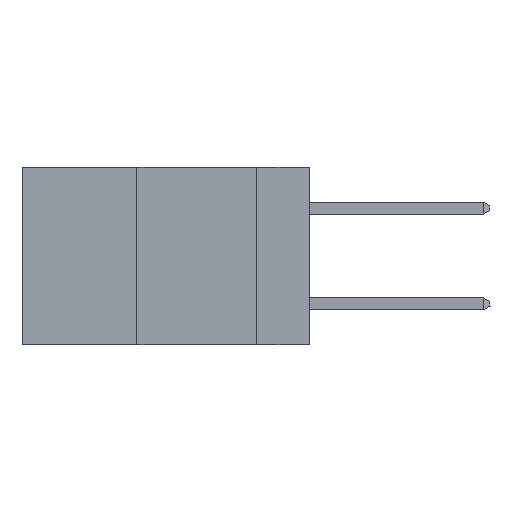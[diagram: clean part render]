
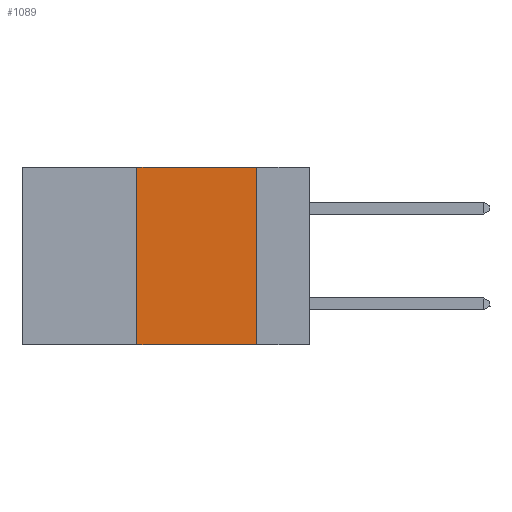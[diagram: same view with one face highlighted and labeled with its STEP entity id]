
A CAD part, left-side view. The second image highlights one B-rep face of the part: STEP entity #1089.
In plain terms, the highlighted planar face has unit normal (-1, 0, 0).
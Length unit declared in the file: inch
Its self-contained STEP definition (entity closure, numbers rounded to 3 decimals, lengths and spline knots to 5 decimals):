
#1089 = ADVANCED_FACE ( 'NONE', ( #18183 ), #6968, .F. ) ;
#2550 = DIRECTION ( 'NONE',  ( 0., 0., -1. ) ) ;
#3402 = DIRECTION ( 'NONE',  ( 0., -1., 0. ) ) ;
#4809 = CARTESIAN_POINT ( 'NONE',  ( 0., 0.6, 0. ) ) ;
#5420 = LINE ( 'NONE', #9949, #6219 ) ;
#6219 = VECTOR ( 'NONE', #8189, 39.37008 ) ;
#6968 = PLANE ( 'NONE',  #12560 ) ;
#7091 = ORIENTED_EDGE ( 'NONE', *, *, #21090, .T. ) ;
#7540 = CARTESIAN_POINT ( 'NONE',  ( 0., 0.36, 0. ) ) ;
#8189 = DIRECTION ( 'NONE',  ( 0., 0., 1. ) ) ;
#8249 = EDGE_CURVE ( 'NONE', #21827, #9109, #5420, .T. ) ;
#8708 = CARTESIAN_POINT ( 'NONE',  ( 0., 0.6, 0. ) ) ;
#9109 = VERTEX_POINT ( 'NONE', #7540 ) ;
#9276 = EDGE_CURVE ( 'NONE', #9109, #13493, #13647, .T. ) ;
#9461 = CARTESIAN_POINT ( 'NONE',  ( 0., 0.11, 0. ) ) ;
#9949 = CARTESIAN_POINT ( 'NONE',  ( 0., 0.36, 0. ) ) ;
#11023 = VECTOR ( 'NONE', #3402, 39.37008 ) ;
#11106 = ORIENTED_EDGE ( 'NONE', *, *, #9276, .F. ) ;
#12333 = VECTOR ( 'NONE', #13307, 39.37008 ) ;
#12560 = AXIS2_PLACEMENT_3D ( 'NONE', #8708, #12609, #2550 ) ;
#12609 = DIRECTION ( 'NONE',  ( 1., 0., 0. ) ) ;
#13307 = DIRECTION ( 'NONE',  ( 0., -1., 0. ) ) ;
#13493 = VERTEX_POINT ( 'NONE', #21792 ) ;
#13608 = CARTESIAN_POINT ( 'NONE',  ( 0., 0.6, -0.37 ) ) ;
#13647 = LINE ( 'NONE', #4809, #12333 ) ;
#14150 = EDGE_LOOP ( 'NONE', ( #15765, #11106, #20544, #7091 ) ) ;
#15549 = LINE ( 'NONE', #13608, #11023 ) ;
#15765 = ORIENTED_EDGE ( 'NONE', *, *, #19233, .F. ) ;
#15912 = CARTESIAN_POINT ( 'NONE',  ( 0., 0.36, -0.37 ) ) ;
#17934 = VERTEX_POINT ( 'NONE', #21008 ) ;
#18183 = FACE_OUTER_BOUND ( 'NONE', #14150, .T. ) ;
#19121 = VECTOR ( 'NONE', #21172, 39.37008 ) ;
#19233 = EDGE_CURVE ( 'NONE', #13493, #17934, #22044, .T. ) ;
#20544 = ORIENTED_EDGE ( 'NONE', *, *, #8249, .F. ) ;
#21008 = CARTESIAN_POINT ( 'NONE',  ( 0., 0.11, -0.37 ) ) ;
#21090 = EDGE_CURVE ( 'NONE', #21827, #17934, #15549, .T. ) ;
#21172 = DIRECTION ( 'NONE',  ( 0., 0., -1. ) ) ;
#21792 = CARTESIAN_POINT ( 'NONE',  ( 0., 0.11, 0. ) ) ;
#21827 = VERTEX_POINT ( 'NONE', #15912 ) ;
#22044 = LINE ( 'NONE', #9461, #19121 ) ;
